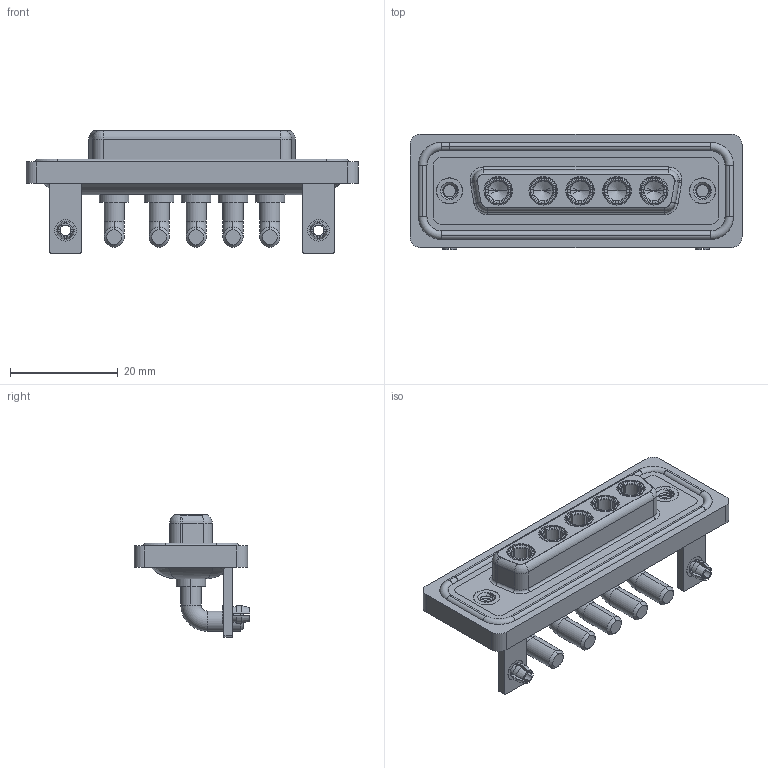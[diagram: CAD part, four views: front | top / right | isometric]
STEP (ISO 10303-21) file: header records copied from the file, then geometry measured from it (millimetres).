
FILE_DESCRIPTION (( 'STEP AP203' ), '1' );
FILE_NAME ('630W5W5-240-4N3.STEP', '2024-04-12T00:21:00', ( '' ), ( '' ), 'SwSTEP 2.0', 'SolidWorks 2023', '' );
FILE_SCHEMA (( 'CONFIG_CONTROL_DESIGN' ));
Length unit declared in the file: millimetre
Products named in the file (9): 630Combo Waterproof Housing_25 Contacts; 630Combo Board Lock_50 Contacts; 630W5W5-240-4N3; 630Combo Stabilizer Bracket_50 Contacts; 630Combo Threaded Rivet_2; Power Socket_40A RA; 630Combo Shell Rear_25 Contacts; 630Combo Housing_5W5; 630Combo Shell Front_25 Contacts
Assembly tree (15 placements, depth 2):
  630W5W5-240-4N3
    630Combo Housing_5W5
    630Combo Shell Front_25 Contacts
    630Combo Shell Rear_25 Contacts
    630Combo Threaded Rivet_2  x2
    630Combo Stabilizer Bracket_50 Contacts  x2
    630Combo Board Lock_50 Contacts  x2
    Power Socket_40A RA  x5
    630Combo Waterproof Housing_25 Contacts
Bounding box: 61.75 x 21.5 x 22.8 mm (x, y, z)
Volume: 9201.5 mm3; surface area: 14977.7 mm2
Topology: 21 solids, 21 shells, 916 faces, 2367 edges, 1515 vertices
Faces by surface type: cylinder 369, plane 318, cone 113, torus 101, bspline 15
Entity records: 18938 total; most frequent: CARTESIAN_POINT 4968, DIRECTION 2836, ORIENTED_EDGE 2632, EDGE_CURVE 1316, AXIS2_PLACEMENT_3D 1130, VERTEX_POINT 841, CIRCLE 599, EDGE_LOOP 579
